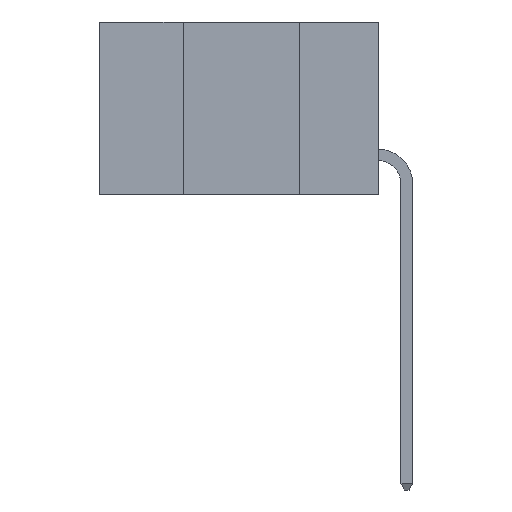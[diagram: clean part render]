
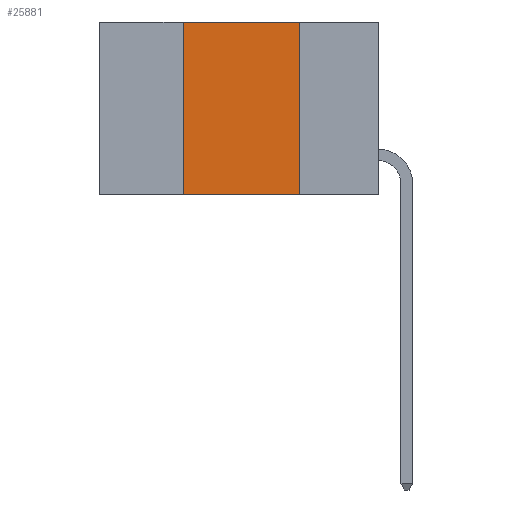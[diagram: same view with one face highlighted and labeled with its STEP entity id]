
A CAD part, left-side view. The second image highlights one B-rep face of the part: STEP entity #25881.
In plain terms, the highlighted planar face has unit normal (-1, 0, 0).
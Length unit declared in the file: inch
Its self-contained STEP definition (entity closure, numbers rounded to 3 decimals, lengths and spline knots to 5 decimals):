
#791 = FACE_OUTER_BOUND ( 'NONE', #20549, .T. ) ;
#1097 = ORIENTED_EDGE ( 'NONE', *, *, #2689, .F. ) ;
#2326 = VECTOR ( 'NONE', #3404, 39.37008 ) ;
#2689 = EDGE_CURVE ( 'NONE', #8061, #25160, #17443, .T. ) ;
#2928 = CARTESIAN_POINT ( 'NONE',  ( 0., 0.17, 0. ) ) ;
#3404 = DIRECTION ( 'NONE',  ( 0., -1., 0. ) ) ;
#3804 = CARTESIAN_POINT ( 'NONE',  ( 0., 0.42, 0. ) ) ;
#3815 = AXIS2_PLACEMENT_3D ( 'NONE', #9461, #23150, #11492 ) ;
#4534 = CARTESIAN_POINT ( 'NONE',  ( 0., 0.42, -0.37 ) ) ;
#5904 = CARTESIAN_POINT ( 'NONE',  ( 0., 0.17, -0.37 ) ) ;
#7919 = ORIENTED_EDGE ( 'NONE', *, *, #8281, .F. ) ;
#8061 = VERTEX_POINT ( 'NONE', #3804 ) ;
#8281 = EDGE_CURVE ( 'NONE', #19042, #8061, #18404, .T. ) ;
#8699 = CARTESIAN_POINT ( 'NONE',  ( 0., 0.42, -0.37 ) ) ;
#9325 = DIRECTION ( 'NONE',  ( 0., -1., 0. ) ) ;
#9461 = CARTESIAN_POINT ( 'NONE',  ( 0., 0.6, 0. ) ) ;
#9773 = CARTESIAN_POINT ( 'NONE',  ( 0., 0.17, -0.37 ) ) ;
#11492 = DIRECTION ( 'NONE',  ( 0., 0., -1. ) ) ;
#11511 = LINE ( 'NONE', #5904, #16147 ) ;
#13654 = CARTESIAN_POINT ( 'NONE',  ( 0., 0.6, -0.37 ) ) ;
#13708 = EDGE_CURVE ( 'NONE', #19042, #22431, #16385, .T. ) ;
#14777 = DIRECTION ( 'NONE',  ( 0., 0., 1. ) ) ;
#15455 = ORIENTED_EDGE ( 'NONE', *, *, #20721, .F. ) ;
#15644 = ORIENTED_EDGE ( 'NONE', *, *, #13708, .T. ) ;
#16147 = VECTOR ( 'NONE', #17993, 39.37008 ) ;
#16385 = LINE ( 'NONE', #13654, #2326 ) ;
#16817 = VECTOR ( 'NONE', #9325, 39.37008 ) ;
#17443 = LINE ( 'NONE', #24804, #16817 ) ;
#17993 = DIRECTION ( 'NONE',  ( 0., 0., -1. ) ) ;
#18404 = LINE ( 'NONE', #8699, #22880 ) ;
#19042 = VERTEX_POINT ( 'NONE', #4534 ) ;
#20549 = EDGE_LOOP ( 'NONE', ( #15455, #1097, #7919, #15644 ) ) ;
#20721 = EDGE_CURVE ( 'NONE', #25160, #22431, #11511, .T. ) ;
#21258 = PLANE ( 'NONE',  #3815 ) ;
#22431 = VERTEX_POINT ( 'NONE', #9773 ) ;
#22880 = VECTOR ( 'NONE', #14777, 39.37008 ) ;
#23150 = DIRECTION ( 'NONE',  ( 1., 0., 0. ) ) ;
#24804 = CARTESIAN_POINT ( 'NONE',  ( 0., 0.6, 0. ) ) ;
#25160 = VERTEX_POINT ( 'NONE', #2928 ) ;
#25881 = ADVANCED_FACE ( 'NONE', ( #791 ), #21258, .F. ) ;
